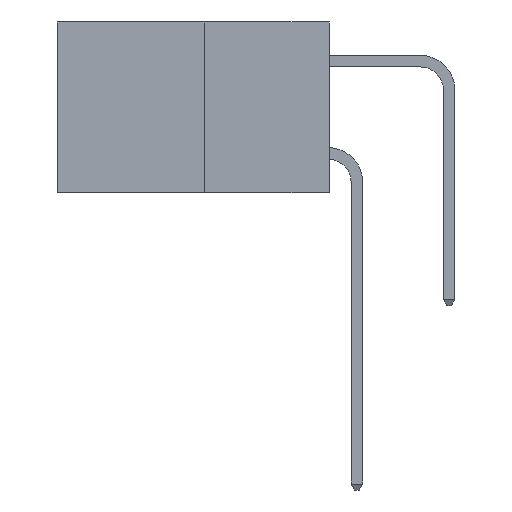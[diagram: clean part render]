
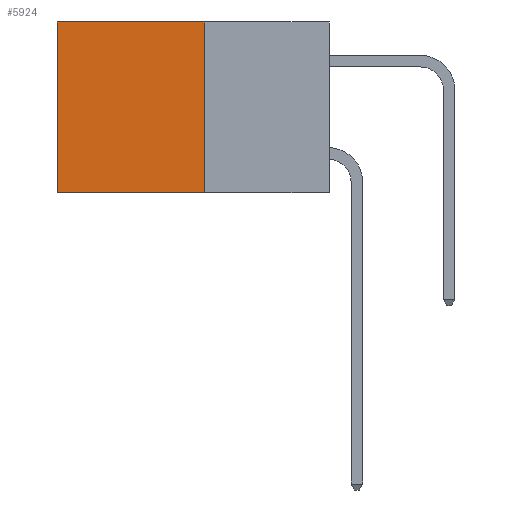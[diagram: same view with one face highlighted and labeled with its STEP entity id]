
A CAD part, left-side view. The second image highlights one B-rep face of the part: STEP entity #5924.
In plain terms, the highlighted planar face has unit normal (-1, 0, 0).
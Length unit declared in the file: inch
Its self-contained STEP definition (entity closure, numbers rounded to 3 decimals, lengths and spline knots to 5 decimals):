
#34 = LINE ( 'NONE', #641, #4063 ) ;
#235 = LINE ( 'NONE', #3228, #7932 ) ;
#386 = VECTOR ( 'NONE', #7275, 39.37008 ) ;
#641 = CARTESIAN_POINT ( 'NONE',  ( 0.277, 0.27, -0.37 ) ) ;
#703 = CARTESIAN_POINT ( 'NONE',  ( 0.277, 0.59, -0.37 ) ) ;
#866 = CARTESIAN_POINT ( 'NONE',  ( 0.277, 0.27, -0.37 ) ) ;
#1168 = PLANE ( 'NONE',  #4788 ) ;
#1911 = ORIENTED_EDGE ( 'NONE', *, *, #8469, .F. ) ;
#2971 = ORIENTED_EDGE ( 'NONE', *, *, #6477, .F. ) ;
#3228 = CARTESIAN_POINT ( 'NONE',  ( 0.277, 0.27, -0.37 ) ) ;
#3687 = LINE ( 'NONE', #4452, #3915 ) ;
#3915 = VECTOR ( 'NONE', #9639, 39.37008 ) ;
#3954 = DIRECTION ( 'NONE',  ( 0., 0., -1. ) ) ;
#4063 = VECTOR ( 'NONE', #6320, 39.37008 ) ;
#4185 = VERTEX_POINT ( 'NONE', #703 ) ;
#4242 = CARTESIAN_POINT ( 'NONE',  ( 0.277, 0.27, -0.37 ) ) ;
#4265 = DIRECTION ( 'NONE',  ( 0., 0., -1. ) ) ;
#4396 = LINE ( 'NONE', #4660, #386 ) ;
#4452 = CARTESIAN_POINT ( 'NONE',  ( 0.277, 0.59, -0.37 ) ) ;
#4660 = CARTESIAN_POINT ( 'NONE',  ( 0.277, 0.27, 0. ) ) ;
#4788 = AXIS2_PLACEMENT_3D ( 'NONE', #4242, #7096, #4265 ) ;
#4953 = ORIENTED_EDGE ( 'NONE', *, *, #6230, .T. ) ;
#5397 = ORIENTED_EDGE ( 'NONE', *, *, #8293, .T. ) ;
#5924 = ADVANCED_FACE ( 'NONE', ( #7012 ), #1168, .F. ) ;
#6230 = EDGE_CURVE ( 'NONE', #6834, #9232, #4396, .T. ) ;
#6273 = CARTESIAN_POINT ( 'NONE',  ( 0.277, 0.59, 0. ) ) ;
#6282 = CARTESIAN_POINT ( 'NONE',  ( 0.277, 0.27, 0. ) ) ;
#6320 = DIRECTION ( 'NONE',  ( 0., 1., 0. ) ) ;
#6477 = EDGE_CURVE ( 'NONE', #6690, #4185, #34, .T. ) ;
#6690 = VERTEX_POINT ( 'NONE', #866 ) ;
#6834 = VERTEX_POINT ( 'NONE', #6282 ) ;
#7012 = FACE_OUTER_BOUND ( 'NONE', #8222, .T. ) ;
#7096 = DIRECTION ( 'NONE',  ( 1., 0., 0. ) ) ;
#7275 = DIRECTION ( 'NONE',  ( 0., 1., 0. ) ) ;
#7932 = VECTOR ( 'NONE', #3954, 39.37008 ) ;
#8222 = EDGE_LOOP ( 'NONE', ( #5397, #2971, #1911, #4953 ) ) ;
#8293 = EDGE_CURVE ( 'NONE', #9232, #4185, #3687, .T. ) ;
#8469 = EDGE_CURVE ( 'NONE', #6834, #6690, #235, .T. ) ;
#9232 = VERTEX_POINT ( 'NONE', #6273 ) ;
#9639 = DIRECTION ( 'NONE',  ( 0., 0., -1. ) ) ;
